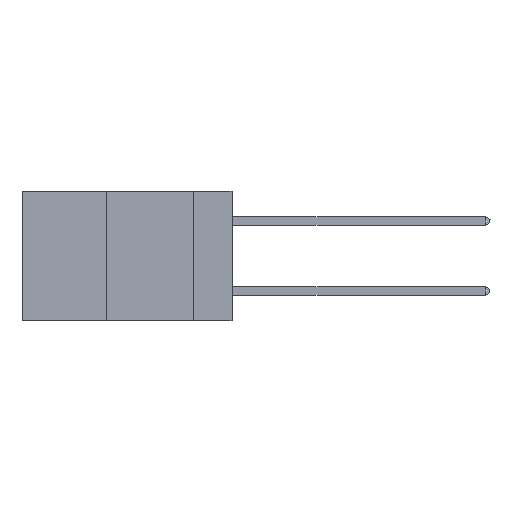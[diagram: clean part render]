
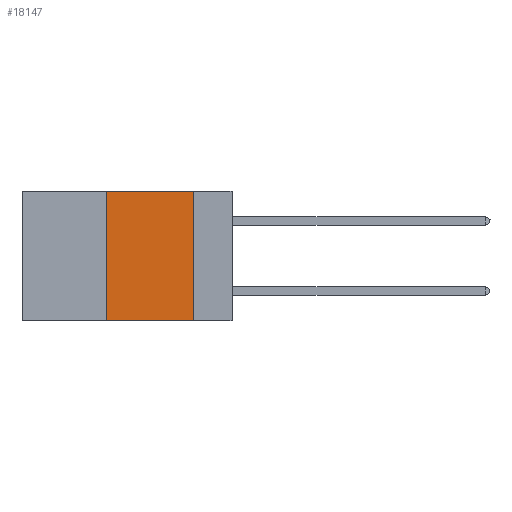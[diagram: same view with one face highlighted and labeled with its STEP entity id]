
A CAD part, left-side view. The second image highlights one B-rep face of the part: STEP entity #18147.
In plain terms, the highlighted planar face has unit normal (-1, 0, 0).
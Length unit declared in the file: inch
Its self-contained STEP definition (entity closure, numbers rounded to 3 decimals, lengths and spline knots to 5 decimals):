
#339 = VERTEX_POINT ( 'NONE', #41798 ) ;
#2863 = DIRECTION ( 'NONE',  ( 0., 0., -1. ) ) ;
#4617 = FACE_OUTER_BOUND ( 'NONE', #23480, .T. ) ;
#7868 = DIRECTION ( 'NONE',  ( 1., 0., 0. ) ) ;
#7874 = ORIENTED_EDGE ( 'NONE', *, *, #16970, .F. ) ;
#8203 = VECTOR ( 'NONE', #15154, 39.37008 ) ;
#8742 = VECTOR ( 'NONE', #45195, 39.37008 ) ;
#10059 = LINE ( 'NONE', #23381, #37937 ) ;
#10104 = LINE ( 'NONE', #34511, #8742 ) ;
#11344 = PLANE ( 'NONE',  #45329 ) ;
#11427 = VERTEX_POINT ( 'NONE', #34484 ) ;
#12688 = ORIENTED_EDGE ( 'NONE', *, *, #22193, .F. ) ;
#14388 = DIRECTION ( 'NONE',  ( 0., 0., -1. ) ) ;
#15154 = DIRECTION ( 'NONE',  ( 0., -1., 0. ) ) ;
#16970 = EDGE_CURVE ( 'NONE', #37961, #34533, #23643, .T. ) ;
#18147 = ADVANCED_FACE ( 'NONE', ( #4617 ), #11344, .F. ) ;
#20157 = CARTESIAN_POINT ( 'NONE',  ( 0., 0.36, 0. ) ) ;
#20733 = EDGE_CURVE ( 'NONE', #37961, #339, #40231, .T. ) ;
#22193 = EDGE_CURVE ( 'NONE', #11427, #339, #10059, .T. ) ;
#23381 = CARTESIAN_POINT ( 'NONE',  ( 0., 0.11, 0. ) ) ;
#23480 = EDGE_LOOP ( 'NONE', ( #12688, #45053, #7874, #43020 ) ) ;
#23643 = LINE ( 'NONE', #20157, #38745 ) ;
#24128 = CARTESIAN_POINT ( 'NONE',  ( 0., 0.36, -0.37 ) ) ;
#26900 = DIRECTION ( 'NONE',  ( 0., 0., 1. ) ) ;
#33495 = CARTESIAN_POINT ( 'NONE',  ( 0., 0.6, -0.37 ) ) ;
#34484 = CARTESIAN_POINT ( 'NONE',  ( 0., 0.11, 0. ) ) ;
#34511 = CARTESIAN_POINT ( 'NONE',  ( 0., 0.6, 0. ) ) ;
#34533 = VERTEX_POINT ( 'NONE', #42936 ) ;
#37937 = VECTOR ( 'NONE', #2863, 39.37008 ) ;
#37961 = VERTEX_POINT ( 'NONE', #24128 ) ;
#38745 = VECTOR ( 'NONE', #26900, 39.37008 ) ;
#39703 = CARTESIAN_POINT ( 'NONE',  ( 0., 0.6, 0. ) ) ;
#40231 = LINE ( 'NONE', #33495, #8203 ) ;
#41345 = EDGE_CURVE ( 'NONE', #34533, #11427, #10104, .T. ) ;
#41798 = CARTESIAN_POINT ( 'NONE',  ( 0., 0.11, -0.37 ) ) ;
#42936 = CARTESIAN_POINT ( 'NONE',  ( 0., 0.36, 0. ) ) ;
#43020 = ORIENTED_EDGE ( 'NONE', *, *, #20733, .T. ) ;
#45053 = ORIENTED_EDGE ( 'NONE', *, *, #41345, .F. ) ;
#45195 = DIRECTION ( 'NONE',  ( 0., -1., 0. ) ) ;
#45329 = AXIS2_PLACEMENT_3D ( 'NONE', #39703, #7868, #14388 ) ;
